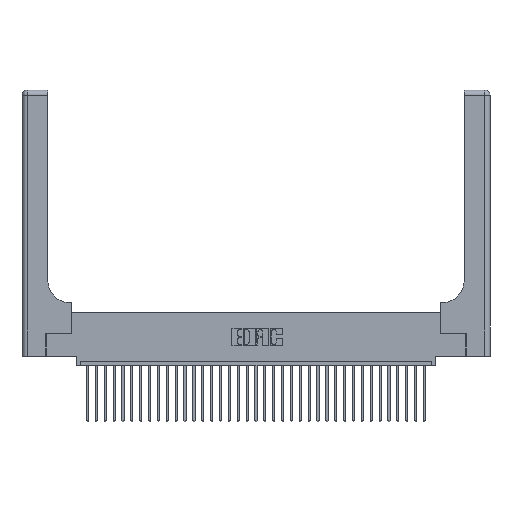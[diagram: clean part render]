
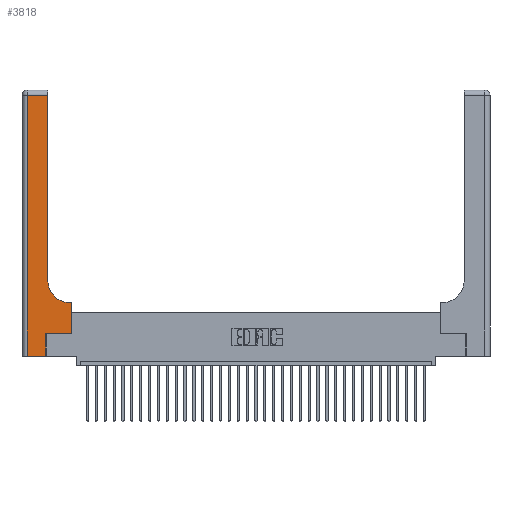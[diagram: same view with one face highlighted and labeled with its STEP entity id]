
A CAD part, top view. The second image highlights one B-rep face of the part: STEP entity #3818.
In plain terms, the highlighted planar face has unit normal (0, 0, 1).
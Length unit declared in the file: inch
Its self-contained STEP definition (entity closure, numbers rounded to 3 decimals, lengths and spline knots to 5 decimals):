
#14 = CARTESIAN_POINT ( 'NONE',  ( 0.269, 0., 0.37 ) ) ;
#849 = VERTEX_POINT ( 'NONE', #22108 ) ;
#1419 = EDGE_CURVE ( 'NONE', #3307, #29919, #2176, .T. ) ;
#2176 = LINE ( 'NONE', #15873, #22930 ) ;
#2709 = EDGE_CURVE ( 'NONE', #849, #7040, #20764, .T. ) ;
#2723 = VERTEX_POINT ( 'NONE', #16276 ) ;
#2916 = CARTESIAN_POINT ( 'NONE',  ( 0.2915, 0.85, 0.37 ) ) ;
#3307 = VERTEX_POINT ( 'NONE', #17793 ) ;
#3818 = ADVANCED_FACE ( 'NONE', ( #11367 ), #7299, .F. ) ;
#4312 = CARTESIAN_POINT ( 'NONE',  ( 0.06, 0., 0.37 ) ) ;
#4851 = VECTOR ( 'NONE', #15247, 39.37008 ) ;
#4876 = DIRECTION ( 'NONE',  ( 1., 0., 0. ) ) ;
#4994 = CARTESIAN_POINT ( 'NONE',  ( 0.06, 2.94, 0.37 ) ) ;
#5081 = EDGE_CURVE ( 'NONE', #21355, #3307, #13456, .T. ) ;
#5460 = ORIENTED_EDGE ( 'NONE', *, *, #5081, .T. ) ;
#5676 = LINE ( 'NONE', #25732, #4851 ) ;
#5932 = ORIENTED_EDGE ( 'NONE', *, *, #1419, .T. ) ;
#6299 = ORIENTED_EDGE ( 'NONE', *, *, #17849, .T. ) ;
#7040 = VERTEX_POINT ( 'NONE', #20052 ) ;
#7061 = CARTESIAN_POINT ( 'NONE',  ( 0., 0., 0.37 ) ) ;
#7299 = PLANE ( 'NONE',  #29790 ) ;
#7674 = CARTESIAN_POINT ( 'NONE',  ( 0.06, 3., 0.37 ) ) ;
#7732 = DIRECTION ( 'NONE',  ( 0., 1., 0. ) ) ;
#10078 = EDGE_CURVE ( 'NONE', #2723, #18650, #5676, .T. ) ;
#10284 = DIRECTION ( 'NONE',  ( 0., -1., 0. ) ) ;
#11367 = FACE_OUTER_BOUND ( 'NONE', #22763, .T. ) ;
#12263 = VECTOR ( 'NONE', #7732, 39.37008 ) ;
#12675 = DIRECTION ( 'NONE',  ( 0., 0., -1. ) ) ;
#12789 = CARTESIAN_POINT ( 'NONE',  ( 0.5585, 0.25, 0.37 ) ) ;
#12864 = VECTOR ( 'NONE', #4876, 39.37008 ) ;
#13184 = EDGE_CURVE ( 'NONE', #29919, #27422, #32230, .T. ) ;
#13456 = LINE ( 'NONE', #25893, #26970 ) ;
#13590 = LINE ( 'NONE', #7674, #20776 ) ;
#14412 = ORIENTED_EDGE ( 'NONE', *, *, #10078, .T. ) ;
#15247 = DIRECTION ( 'NONE',  ( -1., 0., 0. ) ) ;
#15868 = ORIENTED_EDGE ( 'NONE', *, *, #32432, .T. ) ;
#15873 = CARTESIAN_POINT ( 'NONE',  ( 0.2915, 0.6, 0.37 ) ) ;
#16276 = CARTESIAN_POINT ( 'NONE',  ( 0.2915, 2.94, 0.37 ) ) ;
#16733 = LINE ( 'NONE', #7061, #31117 ) ;
#17308 = LINE ( 'NONE', #28289, #23635 ) ;
#17793 = CARTESIAN_POINT ( 'NONE',  ( 0.5585, 0.6, 0.37 ) ) ;
#17849 = EDGE_CURVE ( 'NONE', #18650, #26650, #13590, .T. ) ;
#18494 = ORIENTED_EDGE ( 'NONE', *, *, #21242, .T. ) ;
#18650 = VERTEX_POINT ( 'NONE', #4994 ) ;
#20052 = CARTESIAN_POINT ( 'NONE',  ( 0.269, 0.25, 0.37 ) ) ;
#20134 = DIRECTION ( 'NONE',  ( 0., 1., 0. ) ) ;
#20764 = LINE ( 'NONE', #14, #12263 ) ;
#20776 = VECTOR ( 'NONE', #10284, 39.37008 ) ;
#21242 = EDGE_CURVE ( 'NONE', #26650, #849, #16733, .T. ) ;
#21355 = VERTEX_POINT ( 'NONE', #12789 ) ;
#21714 = DIRECTION ( 'NONE',  ( -1., 0., 0. ) ) ;
#22026 = EDGE_CURVE ( 'NONE', #7040, #21355, #30658, .T. ) ;
#22108 = CARTESIAN_POINT ( 'NONE',  ( 0.269, 0., 0.37 ) ) ;
#22321 = DIRECTION ( 'NONE',  ( 0., 0., -1. ) ) ;
#22763 = EDGE_LOOP ( 'NONE', ( #15868, #14412, #6299, #18494, #25938, #22811, #5460, #5932, #29340 ) ) ;
#22811 = ORIENTED_EDGE ( 'NONE', *, *, #22026, .T. ) ;
#22930 = VECTOR ( 'NONE', #31710, 39.37008 ) ;
#23430 = AXIS2_PLACEMENT_3D ( 'NONE', #23656, #12675, #33956 ) ;
#23635 = VECTOR ( 'NONE', #20134, 39.37008 ) ;
#23656 = CARTESIAN_POINT ( 'NONE',  ( 0.5415, 0.85, 0.37 ) ) ;
#25732 = CARTESIAN_POINT ( 'NONE',  ( 0., 2.94, 0.37 ) ) ;
#25893 = CARTESIAN_POINT ( 'NONE',  ( 0.5585, 0.25, 0.37 ) ) ;
#25938 = ORIENTED_EDGE ( 'NONE', *, *, #2709, .T. ) ;
#26650 = VERTEX_POINT ( 'NONE', #4312 ) ;
#26668 = CARTESIAN_POINT ( 'NONE',  ( 0.269, 0.25, 0.37 ) ) ;
#26970 = VECTOR ( 'NONE', #27253, 39.37008 ) ;
#27253 = DIRECTION ( 'NONE',  ( 0., 1., 0. ) ) ;
#27422 = VERTEX_POINT ( 'NONE', #2916 ) ;
#28289 = CARTESIAN_POINT ( 'NONE',  ( 0.2915, 3., 0.37 ) ) ;
#28764 = DIRECTION ( 'NONE',  ( 1., 0., 0. ) ) ;
#29340 = ORIENTED_EDGE ( 'NONE', *, *, #13184, .T. ) ;
#29790 = AXIS2_PLACEMENT_3D ( 'NONE', #33559, #22321, #21714 ) ;
#29919 = VERTEX_POINT ( 'NONE', #31494 ) ;
#30658 = LINE ( 'NONE', #26668, #12864 ) ;
#31117 = VECTOR ( 'NONE', #28764, 39.37008 ) ;
#31494 = CARTESIAN_POINT ( 'NONE',  ( 0.5415, 0.6, 0.37 ) ) ;
#31710 = DIRECTION ( 'NONE',  ( -1., 0., 0. ) ) ;
#32230 = CIRCLE ( 'NONE', #23430, 0.25 ) ;
#32432 = EDGE_CURVE ( 'NONE', #27422, #2723, #17308, .T. ) ;
#33559 = CARTESIAN_POINT ( 'NONE',  ( 0., 3., 0.37 ) ) ;
#33956 = DIRECTION ( 'NONE',  ( 1., 0., 0. ) ) ;
